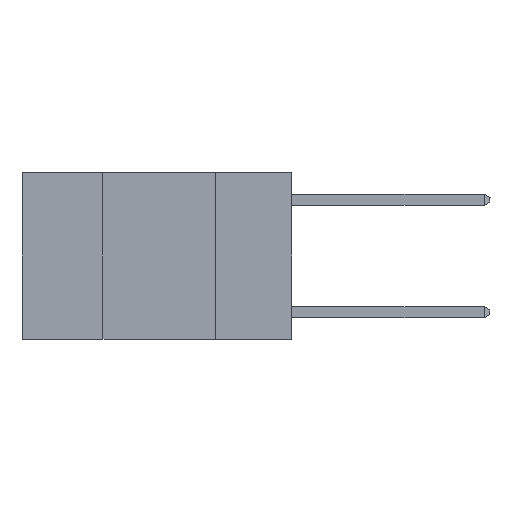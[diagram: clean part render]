
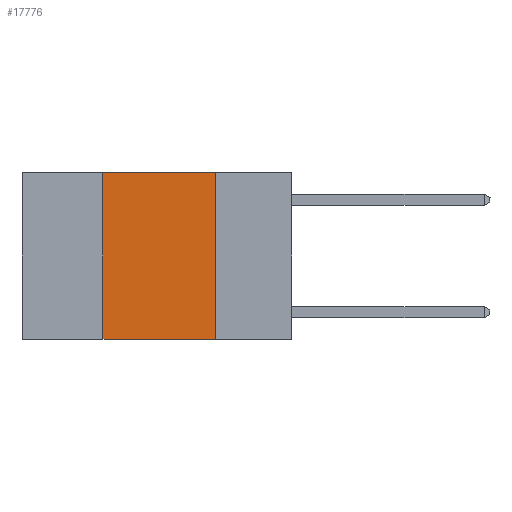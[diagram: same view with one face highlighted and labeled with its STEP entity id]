
A CAD part, left-side view. The second image highlights one B-rep face of the part: STEP entity #17776.
In plain terms, the highlighted planar face has unit normal (-1, 0, 0).
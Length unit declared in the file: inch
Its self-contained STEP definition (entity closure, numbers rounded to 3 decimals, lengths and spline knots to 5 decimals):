
#23 = DIRECTION ( 'NONE',  ( 1., 0., 0. ) ) ;
#1020 = ORIENTED_EDGE ( 'NONE', *, *, #15991, .F. ) ;
#1161 = CARTESIAN_POINT ( 'NONE',  ( 0., 0.6, -0.37 ) ) ;
#1293 = CARTESIAN_POINT ( 'NONE',  ( 0., 0.6, 0. ) ) ;
#2222 = VECTOR ( 'NONE', #4060, 39.37008 ) ;
#2826 = LINE ( 'NONE', #1161, #3204 ) ;
#3066 = FACE_OUTER_BOUND ( 'NONE', #19123, .T. ) ;
#3076 = VERTEX_POINT ( 'NONE', #5220 ) ;
#3204 = VECTOR ( 'NONE', #10847, 39.37008 ) ;
#3754 = ORIENTED_EDGE ( 'NONE', *, *, #19547, .F. ) ;
#4060 = DIRECTION ( 'NONE',  ( 0., 0., -1. ) ) ;
#5102 = ORIENTED_EDGE ( 'NONE', *, *, #14981, .T. ) ;
#5220 = CARTESIAN_POINT ( 'NONE',  ( 0., 0.17, -0.37 ) ) ;
#5545 = CARTESIAN_POINT ( 'NONE',  ( 0., 0.17, 0. ) ) ;
#5978 = LINE ( 'NONE', #7339, #12087 ) ;
#6048 = PLANE ( 'NONE',  #17673 ) ;
#6164 = VERTEX_POINT ( 'NONE', #8014 ) ;
#6876 = DIRECTION ( 'NONE',  ( 0., 0., 1. ) ) ;
#7280 = VERTEX_POINT ( 'NONE', #5545 ) ;
#7339 = CARTESIAN_POINT ( 'NONE',  ( 0., 0.6, 0. ) ) ;
#7624 = DIRECTION ( 'NONE',  ( 0., 0., -1. ) ) ;
#8014 = CARTESIAN_POINT ( 'NONE',  ( 0., 0.42, 0. ) ) ;
#10294 = DIRECTION ( 'NONE',  ( 0., -1., 0. ) ) ;
#10847 = DIRECTION ( 'NONE',  ( 0., -1., 0. ) ) ;
#12032 = LINE ( 'NONE', #16505, #13387 ) ;
#12087 = VECTOR ( 'NONE', #10294, 39.37008 ) ;
#13387 = VECTOR ( 'NONE', #6876, 39.37008 ) ;
#14981 = EDGE_CURVE ( 'NONE', #15535, #3076, #2826, .T. ) ;
#15535 = VERTEX_POINT ( 'NONE', #18572 ) ;
#15991 = EDGE_CURVE ( 'NONE', #7280, #3076, #18447, .T. ) ;
#16308 = ORIENTED_EDGE ( 'NONE', *, *, #20615, .F. ) ;
#16505 = CARTESIAN_POINT ( 'NONE',  ( 0., 0.42, 0. ) ) ;
#17673 = AXIS2_PLACEMENT_3D ( 'NONE', #1293, #23, #7624 ) ;
#17776 = ADVANCED_FACE ( 'NONE', ( #3066 ), #6048, .F. ) ;
#18447 = LINE ( 'NONE', #20237, #2222 ) ;
#18572 = CARTESIAN_POINT ( 'NONE',  ( 0., 0.42, -0.37 ) ) ;
#19123 = EDGE_LOOP ( 'NONE', ( #1020, #16308, #3754, #5102 ) ) ;
#19547 = EDGE_CURVE ( 'NONE', #15535, #6164, #12032, .T. ) ;
#20237 = CARTESIAN_POINT ( 'NONE',  ( 0., 0.17, 0. ) ) ;
#20615 = EDGE_CURVE ( 'NONE', #6164, #7280, #5978, .T. ) ;
